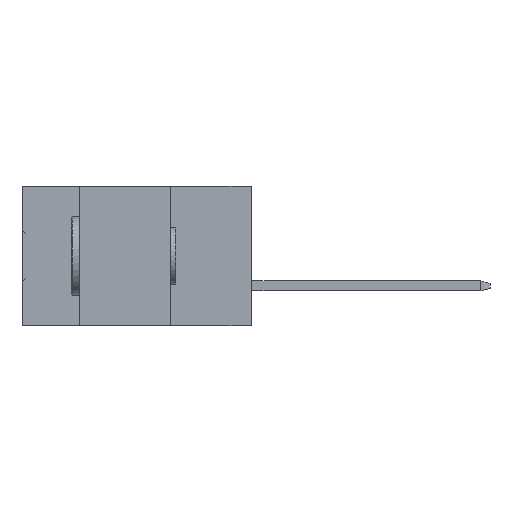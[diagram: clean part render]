
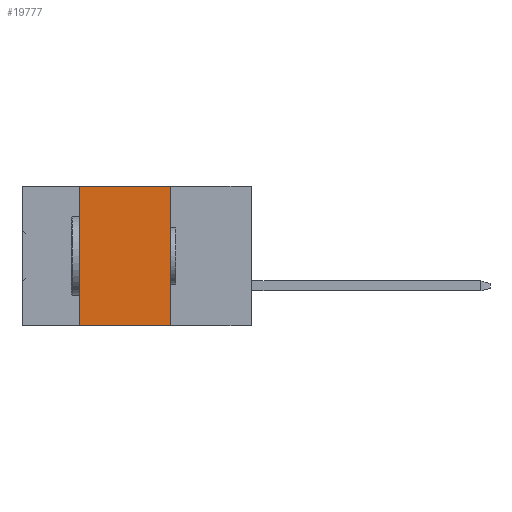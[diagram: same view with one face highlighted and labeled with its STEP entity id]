
A CAD part, left-side view. The second image highlights one B-rep face of the part: STEP entity #19777.
In plain terms, the highlighted planar face has unit normal (-1, 0, 0).
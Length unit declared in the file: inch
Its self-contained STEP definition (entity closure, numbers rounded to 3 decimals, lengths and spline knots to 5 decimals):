
#231 = CARTESIAN_POINT ( 'NONE',  ( 0., 0.54, -0.437 ) ) ;
#1567 = CARTESIAN_POINT ( 'NONE',  ( 0., 0.254, 0. ) ) ;
#1579 = VERTEX_POINT ( 'NONE', #3214 ) ;
#2402 = CARTESIAN_POINT ( 'NONE',  ( 0., 0.254, -0.437 ) ) ;
#2541 = VECTOR ( 'NONE', #5259, 39.37008 ) ;
#2876 = DIRECTION ( 'NONE',  ( 0., -1., 0. ) ) ;
#3214 = CARTESIAN_POINT ( 'NONE',  ( 0., 0.54, -0.437 ) ) ;
#4337 = DIRECTION ( 'NONE',  ( 0., 0., -1. ) ) ;
#5042 = EDGE_CURVE ( 'NONE', #1579, #5056, #22575, .T. ) ;
#5056 = VERTEX_POINT ( 'NONE', #14290 ) ;
#5137 = CARTESIAN_POINT ( 'NONE',  ( 0., 0.72, 0. ) ) ;
#5259 = DIRECTION ( 'NONE',  ( 0., 0., -1. ) ) ;
#5568 = ORIENTED_EDGE ( 'NONE', *, *, #10548, .F. ) ;
#6460 = VECTOR ( 'NONE', #18721, 39.37008 ) ;
#7197 = EDGE_CURVE ( 'NONE', #15713, #5056, #14215, .T. ) ;
#7414 = LINE ( 'NONE', #5137, #8967 ) ;
#8967 = VECTOR ( 'NONE', #2876, 39.37008 ) ;
#9012 = DIRECTION ( 'NONE',  ( 1., 0., 0. ) ) ;
#10548 = EDGE_CURVE ( 'NONE', #1579, #13010, #25651, .T. ) ;
#10578 = ORIENTED_EDGE ( 'NONE', *, *, #5042, .T. ) ;
#13010 = VERTEX_POINT ( 'NONE', #15430 ) ;
#13531 = EDGE_CURVE ( 'NONE', #13010, #15713, #7414, .T. ) ;
#14215 = LINE ( 'NONE', #2402, #2541 ) ;
#14290 = CARTESIAN_POINT ( 'NONE',  ( 0., 0.254, -0.437 ) ) ;
#15430 = CARTESIAN_POINT ( 'NONE',  ( 0., 0.54, 0. ) ) ;
#15713 = VERTEX_POINT ( 'NONE', #1567 ) ;
#18721 = DIRECTION ( 'NONE',  ( 0., 0., 1. ) ) ;
#19777 = ADVANCED_FACE ( 'NONE', ( #25208 ), #22642, .F. ) ;
#20530 = CARTESIAN_POINT ( 'NONE',  ( 0., 0.72, 0. ) ) ;
#20739 = EDGE_LOOP ( 'NONE', ( #21396, #24225, #5568, #10578 ) ) ;
#21396 = ORIENTED_EDGE ( 'NONE', *, *, #7197, .F. ) ;
#22227 = AXIS2_PLACEMENT_3D ( 'NONE', #20530, #9012, #4337 ) ;
#22575 = LINE ( 'NONE', #29503, #26570 ) ;
#22642 = PLANE ( 'NONE',  #22227 ) ;
#24225 = ORIENTED_EDGE ( 'NONE', *, *, #13531, .F. ) ;
#25208 = FACE_OUTER_BOUND ( 'NONE', #20739, .T. ) ;
#25651 = LINE ( 'NONE', #231, #6460 ) ;
#26570 = VECTOR ( 'NONE', #29802, 39.37008 ) ;
#29503 = CARTESIAN_POINT ( 'NONE',  ( 0., 0.72, -0.437 ) ) ;
#29802 = DIRECTION ( 'NONE',  ( 0., -1., 0. ) ) ;
